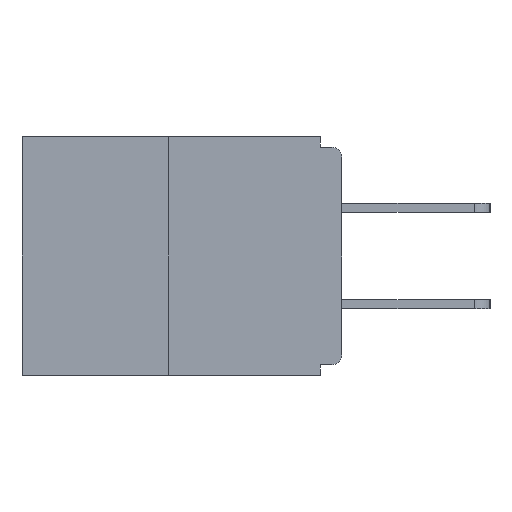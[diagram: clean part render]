
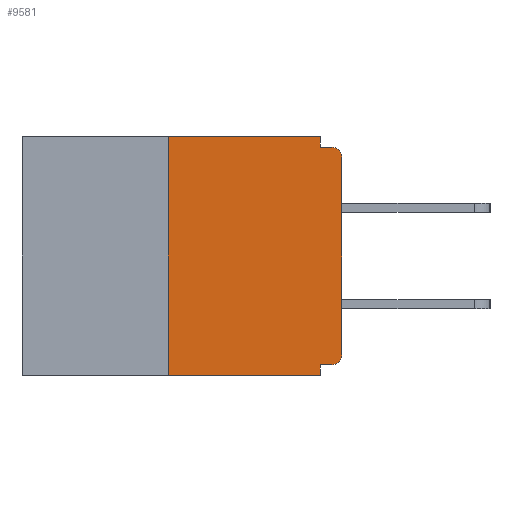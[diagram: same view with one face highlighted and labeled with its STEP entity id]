
A CAD part, left-side view. The second image highlights one B-rep face of the part: STEP entity #9581.
In plain terms, the highlighted planar face has unit normal (-1, 0, 0).
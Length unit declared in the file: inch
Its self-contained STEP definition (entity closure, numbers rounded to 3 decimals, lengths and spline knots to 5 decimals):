
#197 = EDGE_CURVE ( 'NONE', #23367, #836, #14411, .T. ) ;
#224 = CARTESIAN_POINT ( 'NONE',  ( 0., 0., -0.313 ) ) ;
#363 = VECTOR ( 'NONE', #17204, 39.37008 ) ;
#504 = VERTEX_POINT ( 'NONE', #224 ) ;
#690 = CARTESIAN_POINT ( 'NONE',  ( 0., 0.031, 0. ) ) ;
#795 = EDGE_LOOP ( 'NONE', ( #14594, #18947, #16322, #23787, #1013, #23427, #23824, #9325, #22763, #12568 ) ) ;
#836 = VERTEX_POINT ( 'NONE', #22988 ) ;
#1013 = ORIENTED_EDGE ( 'NONE', *, *, #197, .F. ) ;
#1665 = VERTEX_POINT ( 'NONE', #22184 ) ;
#1714 = VERTEX_POINT ( 'NONE', #11426 ) ;
#2464 = FACE_OUTER_BOUND ( 'NONE', #795, .T. ) ;
#2952 = CARTESIAN_POINT ( 'NONE',  ( 0., 0.46, 0. ) ) ;
#3042 = LINE ( 'NONE', #690, #20116 ) ;
#3915 = CARTESIAN_POINT ( 'NONE',  ( 0., 0., -0.03 ) ) ;
#4339 = EDGE_CURVE ( 'NONE', #1714, #18536, #15777, .T. ) ;
#4495 = AXIS2_PLACEMENT_3D ( 'NONE', #12553, #20182, #21940 ) ;
#4640 = DIRECTION ( 'NONE',  ( -1., 0., 0. ) ) ;
#5273 = DIRECTION ( 'NONE',  ( 0., 0., 1. ) ) ;
#5494 = LINE ( 'NONE', #5734, #19655 ) ;
#5562 = EDGE_CURVE ( 'NONE', #9536, #1665, #7716, .T. ) ;
#5734 = CARTESIAN_POINT ( 'NONE',  ( 0., 0.031, -0.343 ) ) ;
#5917 = EDGE_CURVE ( 'NONE', #10178, #1714, #6767, .T. ) ;
#5989 = VECTOR ( 'NONE', #19779, 39.37008 ) ;
#6348 = CARTESIAN_POINT ( 'NONE',  ( 0., 0.031, 0. ) ) ;
#6767 = LINE ( 'NONE', #20122, #9920 ) ;
#7157 = DIRECTION ( 'NONE',  ( 0., -1., 0. ) ) ;
#7202 = CARTESIAN_POINT ( 'NONE',  ( 0., 0.031, -0.015 ) ) ;
#7716 = LINE ( 'NONE', #11217, #363 ) ;
#8040 = CARTESIAN_POINT ( 'NONE',  ( 0., 0.46, 0. ) ) ;
#8360 = CARTESIAN_POINT ( 'NONE',  ( 0., 0.015, -0.313 ) ) ;
#8623 = VERTEX_POINT ( 'NONE', #3915 ) ;
#9033 = EDGE_CURVE ( 'NONE', #836, #14465, #5494, .T. ) ;
#9325 = ORIENTED_EDGE ( 'NONE', *, *, #17418, .T. ) ;
#9536 = VERTEX_POINT ( 'NONE', #7202 ) ;
#9581 = ADVANCED_FACE ( 'NONE', ( #2464 ), #11789, .F. ) ;
#9920 = VECTOR ( 'NONE', #5273, 39.37008 ) ;
#10007 = CARTESIAN_POINT ( 'NONE',  ( 0., 0.031, -0.343 ) ) ;
#10043 = DIRECTION ( 'NONE',  ( 1., 0., 0. ) ) ;
#10178 = VERTEX_POINT ( 'NONE', #23533 ) ;
#10208 = DIRECTION ( 'NONE',  ( 0., 0., 1. ) ) ;
#10500 = EDGE_CURVE ( 'NONE', #10178, #14465, #24527, .T. ) ;
#10554 = CARTESIAN_POINT ( 'NONE',  ( 0., 0., -0.328 ) ) ;
#10698 = CIRCLE ( 'NONE', #23485, 0.015 ) ;
#11217 = CARTESIAN_POINT ( 'NONE',  ( 0., 0., -0.015 ) ) ;
#11426 = CARTESIAN_POINT ( 'NONE',  ( 0., 0.25, 0. ) ) ;
#11789 = PLANE ( 'NONE',  #16489 ) ;
#12200 = EDGE_CURVE ( 'NONE', #23367, #504, #10698, .T. ) ;
#12553 = CARTESIAN_POINT ( 'NONE',  ( 0., 0.015, -0.03 ) ) ;
#12568 = ORIENTED_EDGE ( 'NONE', *, *, #16383, .F. ) ;
#13328 = DIRECTION ( 'NONE',  ( 0., 0., -1. ) ) ;
#13698 = VECTOR ( 'NONE', #7157, 39.37008 ) ;
#14411 = LINE ( 'NONE', #10554, #15778 ) ;
#14465 = VERTEX_POINT ( 'NONE', #10007 ) ;
#14594 = ORIENTED_EDGE ( 'NONE', *, *, #4339, .F. ) ;
#15250 = CIRCLE ( 'NONE', #4495, 0.015 ) ;
#15777 = LINE ( 'NONE', #2952, #5989 ) ;
#15778 = VECTOR ( 'NONE', #23440, 39.37008 ) ;
#16092 = CARTESIAN_POINT ( 'NONE',  ( 0., 0.015, -0.328 ) ) ;
#16322 = ORIENTED_EDGE ( 'NONE', *, *, #10500, .T. ) ;
#16383 = EDGE_CURVE ( 'NONE', #18536, #9536, #3042, .T. ) ;
#16489 = AXIS2_PLACEMENT_3D ( 'NONE', #8040, #10043, #19295 ) ;
#17204 = DIRECTION ( 'NONE',  ( 0., -1., 0. ) ) ;
#17418 = EDGE_CURVE ( 'NONE', #8623, #1665, #15250, .T. ) ;
#17955 = CARTESIAN_POINT ( 'NONE',  ( 0., 0., 0. ) ) ;
#18526 = CARTESIAN_POINT ( 'NONE',  ( 0., 0.46, -0.343 ) ) ;
#18536 = VERTEX_POINT ( 'NONE', #6348 ) ;
#18947 = ORIENTED_EDGE ( 'NONE', *, *, #5917, .F. ) ;
#19295 = DIRECTION ( 'NONE',  ( 0., 0., -1. ) ) ;
#19655 = VECTOR ( 'NONE', #13328, 39.37008 ) ;
#19779 = DIRECTION ( 'NONE',  ( 0., -1., 0. ) ) ;
#19824 = LINE ( 'NONE', #17955, #20548 ) ;
#19991 = DIRECTION ( 'NONE',  ( 0., 0., -1. ) ) ;
#20027 = EDGE_CURVE ( 'NONE', #504, #8623, #19824, .T. ) ;
#20116 = VECTOR ( 'NONE', #19991, 39.37008 ) ;
#20122 = CARTESIAN_POINT ( 'NONE',  ( 0., 0.25, 0. ) ) ;
#20182 = DIRECTION ( 'NONE',  ( -1., 0., 0. ) ) ;
#20548 = VECTOR ( 'NONE', #10208, 39.37008 ) ;
#21940 = DIRECTION ( 'NONE',  ( 0., 0., -1. ) ) ;
#22184 = CARTESIAN_POINT ( 'NONE',  ( 0., 0.015, -0.015 ) ) ;
#22763 = ORIENTED_EDGE ( 'NONE', *, *, #5562, .F. ) ;
#22988 = CARTESIAN_POINT ( 'NONE',  ( 0., 0.031, -0.328 ) ) ;
#23367 = VERTEX_POINT ( 'NONE', #16092 ) ;
#23427 = ORIENTED_EDGE ( 'NONE', *, *, #12200, .T. ) ;
#23440 = DIRECTION ( 'NONE',  ( 0., 1., 0. ) ) ;
#23485 = AXIS2_PLACEMENT_3D ( 'NONE', #8360, #4640, #23615 ) ;
#23533 = CARTESIAN_POINT ( 'NONE',  ( 0., 0.25, -0.343 ) ) ;
#23615 = DIRECTION ( 'NONE',  ( 0., 0., -1. ) ) ;
#23787 = ORIENTED_EDGE ( 'NONE', *, *, #9033, .F. ) ;
#23824 = ORIENTED_EDGE ( 'NONE', *, *, #20027, .T. ) ;
#24527 = LINE ( 'NONE', #18526, #13698 ) ;
